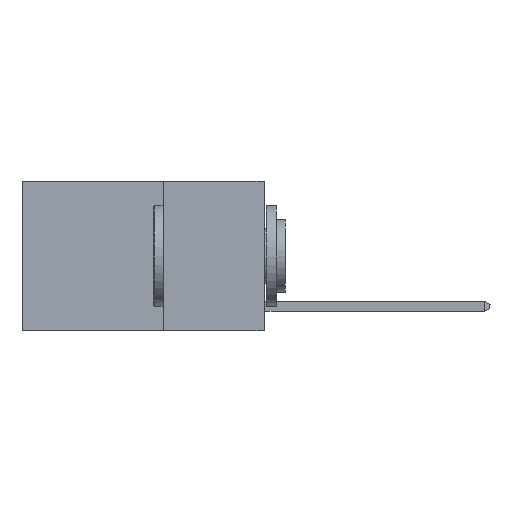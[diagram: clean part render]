
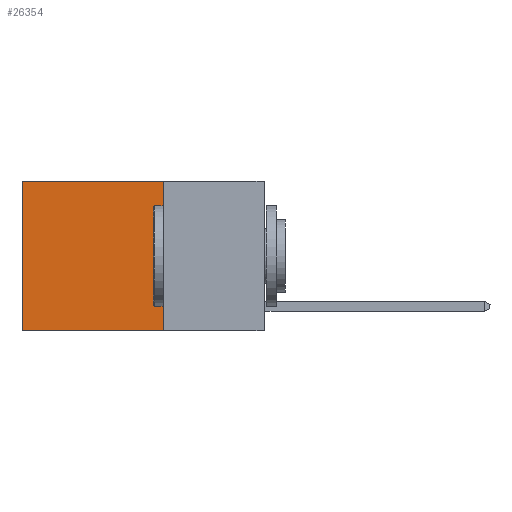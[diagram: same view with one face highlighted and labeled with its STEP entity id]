
A CAD part, left-side view. The second image highlights one B-rep face of the part: STEP entity #26354.
In plain terms, the highlighted planar face has unit normal (-1, 0, 0).
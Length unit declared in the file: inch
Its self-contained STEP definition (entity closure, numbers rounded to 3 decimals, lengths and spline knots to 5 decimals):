
#161 = LINE ( 'NONE', #10571, #7542 ) ;
#1034 = ORIENTED_EDGE ( 'NONE', *, *, #17305, .F. ) ;
#2297 = CARTESIAN_POINT ( 'NONE',  ( 0.2625, 0.6, 0. ) ) ;
#4199 = CARTESIAN_POINT ( 'NONE',  ( 0.2625, 0.25, 0. ) ) ;
#5859 = CARTESIAN_POINT ( 'NONE',  ( 0.2625, 0.6, -0.37 ) ) ;
#6255 = DIRECTION ( 'NONE',  ( 0., 1., 0. ) ) ;
#6693 = DIRECTION ( 'NONE',  ( 1., 0., 0. ) ) ;
#7388 = VECTOR ( 'NONE', #24183, 39.37008 ) ;
#7542 = VECTOR ( 'NONE', #6255, 39.37008 ) ;
#7942 = VERTEX_POINT ( 'NONE', #15002 ) ;
#9242 = CARTESIAN_POINT ( 'NONE',  ( 0.2625, 0.25, 0. ) ) ;
#10571 = CARTESIAN_POINT ( 'NONE',  ( 0.2625, 0.25, -0.37 ) ) ;
#11111 = DIRECTION ( 'NONE',  ( 0., 0., -1. ) ) ;
#12519 = VECTOR ( 'NONE', #28299, 39.37008 ) ;
#13192 = ORIENTED_EDGE ( 'NONE', *, *, #22110, .T. ) ;
#15002 = CARTESIAN_POINT ( 'NONE',  ( 0.2625, 0.25, -0.37 ) ) ;
#15335 = AXIS2_PLACEMENT_3D ( 'NONE', #9242, #6693, #11111 ) ;
#17305 = EDGE_CURVE ( 'NONE', #7942, #18832, #161, .T. ) ;
#17844 = CARTESIAN_POINT ( 'NONE',  ( 0.2625, 0.25, 0. ) ) ;
#18832 = VERTEX_POINT ( 'NONE', #5859 ) ;
#19022 = EDGE_CURVE ( 'NONE', #24305, #18832, #19410, .T. ) ;
#19224 = CARTESIAN_POINT ( 'NONE',  ( 0.2625, 0.25, 0. ) ) ;
#19410 = LINE ( 'NONE', #2297, #23992 ) ;
#19718 = LINE ( 'NONE', #4199, #7388 ) ;
#19732 = CARTESIAN_POINT ( 'NONE',  ( 0.2625, 0.6, 0. ) ) ;
#22110 = EDGE_CURVE ( 'NONE', #24516, #24305, #19718, .T. ) ;
#22122 = ORIENTED_EDGE ( 'NONE', *, *, #19022, .T. ) ;
#22248 = ORIENTED_EDGE ( 'NONE', *, *, #24883, .F. ) ;
#22489 = DIRECTION ( 'NONE',  ( 0., 0., -1. ) ) ;
#23992 = VECTOR ( 'NONE', #22489, 39.37008 ) ;
#24183 = DIRECTION ( 'NONE',  ( 0., 1., 0. ) ) ;
#24305 = VERTEX_POINT ( 'NONE', #19732 ) ;
#24516 = VERTEX_POINT ( 'NONE', #17844 ) ;
#24709 = PLANE ( 'NONE',  #15335 ) ;
#24883 = EDGE_CURVE ( 'NONE', #24516, #7942, #28376, .T. ) ;
#26354 = ADVANCED_FACE ( 'NONE', ( #28926 ), #24709, .F. ) ;
#28299 = DIRECTION ( 'NONE',  ( 0., 0., -1. ) ) ;
#28376 = LINE ( 'NONE', #19224, #12519 ) ;
#28703 = EDGE_LOOP ( 'NONE', ( #22122, #1034, #22248, #13192 ) ) ;
#28926 = FACE_OUTER_BOUND ( 'NONE', #28703, .T. ) ;
